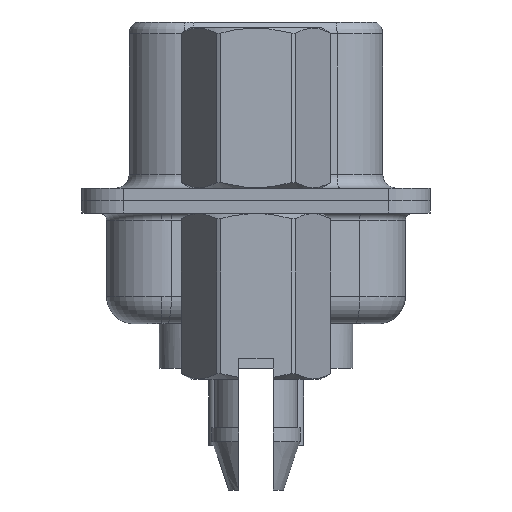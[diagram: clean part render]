
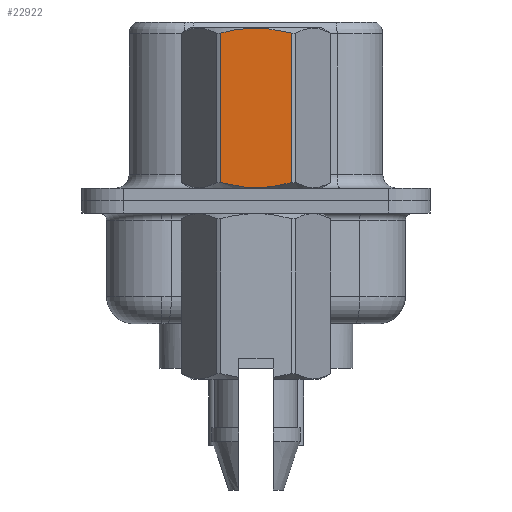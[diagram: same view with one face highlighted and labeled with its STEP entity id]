
A CAD part, left-side view. The second image highlights one B-rep face of the part: STEP entity #22922.
In plain terms, the highlighted planar face has unit normal (-1, 0, 0).
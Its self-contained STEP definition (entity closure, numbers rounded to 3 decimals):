
#547 = CARTESIAN_POINT ( 'NONE',  ( -2.381, -0.215, 0.468 ) ) ;
#571 = CARTESIAN_POINT ( 'NONE',  ( -2.381, 1.273, 3.792 ) ) ;
#816 = EDGE_CURVE ( 'NONE', #17922, #21135, #1331, .T. ) ;
#1331 = B_SPLINE_CURVE_WITH_KNOTS ( 'NONE', 3,
 ( #10651, #17605, #17974, #17515, #10588, #10684, #6283, #5747, #5756, #16186 ),
 .UNSPECIFIED., .F., .F.,
 ( 4, 2, 2, 2, 4 ),
 ( 0.001, 0.002, 0.002, 0.003, 0.004 ),
 .UNSPECIFIED. ) ;
#2641 = CARTESIAN_POINT ( 'NONE',  ( -2.381, -0.858, 0.55 ) ) ;
#3084 = VECTOR ( 'NONE', #19537, 1000. ) ;
#4652 = CARTESIAN_POINT ( 'NONE',  ( -2.381, 1.065, 0.596 ) ) ;
#4755 = CARTESIAN_POINT ( 'NONE',  ( -2.381, -1.273, 0.652 ) ) ;
#5747 = CARTESIAN_POINT ( 'NONE',  ( -2.381, 0.853, 6.151 ) ) ;
#5756 = CARTESIAN_POINT ( 'NONE',  ( -2.381, 1.065, 6.104 ) ) ;
#5800 = FACE_OUTER_BOUND ( 'NONE', #22186, .T. ) ;
#6233 = CARTESIAN_POINT ( 'NONE',  ( -2.381, -1.273, 3.792 ) ) ;
#6283 = CARTESIAN_POINT ( 'NONE',  ( -2.381, 0.428, 6.215 ) ) ;
#6863 = PLANE ( 'NONE',  #14235 ) ;
#6866 = CARTESIAN_POINT ( 'NONE',  ( -2.381, 1.273, 0.652 ) ) ;
#7810 = VECTOR ( 'NONE', #23065, 1000. ) ;
#9009 = DIRECTION ( 'NONE',  ( -1., 0., 0. ) ) ;
#9775 = LINE ( 'NONE', #6233, #7810 ) ;
#10588 = CARTESIAN_POINT ( 'NONE',  ( -2.381, -0.215, 6.232 ) ) ;
#10651 = CARTESIAN_POINT ( 'NONE',  ( -2.381, -1.273, 6.048 ) ) ;
#10684 = CARTESIAN_POINT ( 'NONE',  ( -2.381, 0.215, 6.232 ) ) ;
#11103 = CARTESIAN_POINT ( 'NONE',  ( -2.381, 0.853, 0.549 ) ) ;
#13157 = CARTESIAN_POINT ( 'NONE',  ( -2.381, 0.215, 0.468 ) ) ;
#13592 = ORIENTED_EDGE ( 'NONE', *, *, #24288, .T. ) ;
#14235 = AXIS2_PLACEMENT_3D ( 'NONE', #21553, #9009, #23645 ) ;
#14436 = CARTESIAN_POINT ( 'NONE',  ( -2.381, 1.273, 0.652 ) ) ;
#15266 = CARTESIAN_POINT ( 'NONE',  ( -2.381, -0.432, 0.485 ) ) ;
#16186 = CARTESIAN_POINT ( 'NONE',  ( -2.381, 1.273, 6.048 ) ) ;
#16503 = B_SPLINE_CURVE_WITH_KNOTS ( 'NONE', 3,
 ( #6866, #4652, #11103, #25784, #13157, #547, #15266, #2641, #17373, #4755 ),
 .UNSPECIFIED., .F., .F.,
 ( 4, 2, 2, 2, 4 ),
 ( 0.003, 0.003, 0.004, 0.004, 0.005 ),
 .UNSPECIFIED. ) ;
#17373 = CARTESIAN_POINT ( 'NONE',  ( -2.381, -1.066, 0.596 ) ) ;
#17515 = CARTESIAN_POINT ( 'NONE',  ( -2.381, -0.432, 6.215 ) ) ;
#17605 = CARTESIAN_POINT ( 'NONE',  ( -2.381, -1.066, 6.104 ) ) ;
#17922 = VERTEX_POINT ( 'NONE', #19500 ) ;
#17974 = CARTESIAN_POINT ( 'NONE',  ( -2.381, -0.858, 6.15 ) ) ;
#19185 = ORIENTED_EDGE ( 'NONE', *, *, #21629, .T. ) ;
#19500 = CARTESIAN_POINT ( 'NONE',  ( -2.381, -1.273, 6.048 ) ) ;
#19537 = DIRECTION ( 'NONE',  ( 0., 0., -1. ) ) ;
#19561 = CARTESIAN_POINT ( 'NONE',  ( -2.381, -1.273, 0.652 ) ) ;
#19907 = LINE ( 'NONE', #571, #3084 ) ;
#21135 = VERTEX_POINT ( 'NONE', #25104 ) ;
#21553 = CARTESIAN_POINT ( 'NONE',  ( -2.381, 1.375, -3.75 ) ) ;
#21629 = EDGE_CURVE ( 'NONE', #23443, #17922, #9775, .T. ) ;
#21762 = EDGE_CURVE ( 'NONE', #21135, #24107, #19907, .T. ) ;
#22186 = EDGE_LOOP ( 'NONE', ( #13592, #19185, #23378, #27230 ) ) ;
#22922 = ADVANCED_FACE ( 'NONE', ( #5800 ), #6863, .T. ) ;
#23065 = DIRECTION ( 'NONE',  ( 0., 0., 1. ) ) ;
#23378 = ORIENTED_EDGE ( 'NONE', *, *, #816, .T. ) ;
#23443 = VERTEX_POINT ( 'NONE', #19561 ) ;
#23645 = DIRECTION ( 'NONE',  ( 0., -1., 0. ) ) ;
#24107 = VERTEX_POINT ( 'NONE', #14436 ) ;
#24288 = EDGE_CURVE ( 'NONE', #24107, #23443, #16503, .T. ) ;
#25104 = CARTESIAN_POINT ( 'NONE',  ( -2.381, 1.273, 6.048 ) ) ;
#25784 = CARTESIAN_POINT ( 'NONE',  ( -2.381, 0.428, 0.485 ) ) ;
#27230 = ORIENTED_EDGE ( 'NONE', *, *, #21762, .T. ) ;
